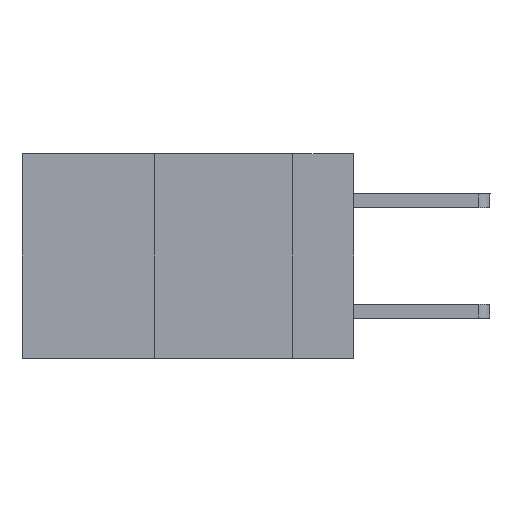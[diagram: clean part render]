
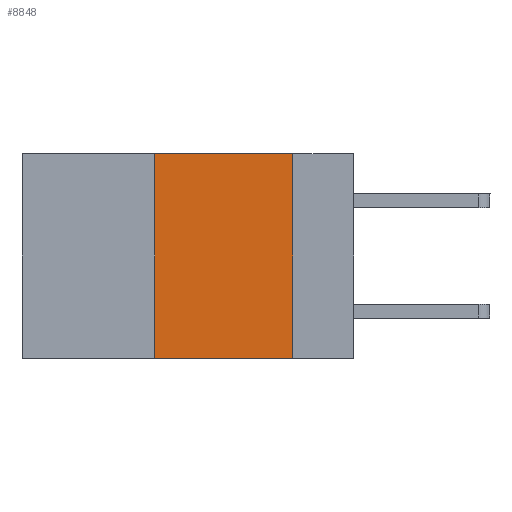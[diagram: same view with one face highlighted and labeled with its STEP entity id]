
A CAD part, left-side view. The second image highlights one B-rep face of the part: STEP entity #8848.
In plain terms, the highlighted planar face has unit normal (-1, 0, 0).
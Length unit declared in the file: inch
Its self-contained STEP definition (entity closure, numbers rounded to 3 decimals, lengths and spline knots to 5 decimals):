
#62 = VERTEX_POINT ( 'NONE', #6391 ) ;
#163 = DIRECTION ( 'NONE',  ( 0., 0., -1. ) ) ;
#187 = VECTOR ( 'NONE', #2608, 39.37008 ) ;
#459 = EDGE_LOOP ( 'NONE', ( #4697, #1227, #5542, #6564 ) ) ;
#501 = CARTESIAN_POINT ( 'NONE',  ( 0., 0.6, 0. ) ) ;
#928 = VERTEX_POINT ( 'NONE', #7984 ) ;
#1227 = ORIENTED_EDGE ( 'NONE', *, *, #7827, .F. ) ;
#1350 = VECTOR ( 'NONE', #163, 39.37008 ) ;
#1680 = CARTESIAN_POINT ( 'NONE',  ( 0., 0.6, -0.37 ) ) ;
#1956 = LINE ( 'NONE', #11112, #2784 ) ;
#2010 = CARTESIAN_POINT ( 'NONE',  ( 0., 0.36, 0. ) ) ;
#2598 = EDGE_CURVE ( 'NONE', #4305, #928, #8859, .T. ) ;
#2608 = DIRECTION ( 'NONE',  ( 0., -1., 0. ) ) ;
#2784 = VECTOR ( 'NONE', #6315, 39.37008 ) ;
#3645 = CARTESIAN_POINT ( 'NONE',  ( 0., 0.11, 0. ) ) ;
#3833 = PLANE ( 'NONE',  #4348 ) ;
#4013 = EDGE_CURVE ( 'NONE', #4519, #928, #6208, .T. ) ;
#4305 = VERTEX_POINT ( 'NONE', #5238 ) ;
#4348 = AXIS2_PLACEMENT_3D ( 'NONE', #501, #10348, #11075 ) ;
#4519 = VERTEX_POINT ( 'NONE', #9901 ) ;
#4697 = ORIENTED_EDGE ( 'NONE', *, *, #2598, .F. ) ;
#5238 = CARTESIAN_POINT ( 'NONE',  ( 0., 0.11, 0. ) ) ;
#5507 = DIRECTION ( 'NONE',  ( 0., 0., 1. ) ) ;
#5542 = ORIENTED_EDGE ( 'NONE', *, *, #11541, .F. ) ;
#6208 = LINE ( 'NONE', #1680, #187 ) ;
#6315 = DIRECTION ( 'NONE',  ( 0., -1., 0. ) ) ;
#6391 = CARTESIAN_POINT ( 'NONE',  ( 0., 0.36, 0. ) ) ;
#6564 = ORIENTED_EDGE ( 'NONE', *, *, #4013, .T. ) ;
#7827 = EDGE_CURVE ( 'NONE', #62, #4305, #1956, .T. ) ;
#7984 = CARTESIAN_POINT ( 'NONE',  ( 0., 0.11, -0.37 ) ) ;
#8111 = LINE ( 'NONE', #2010, #10087 ) ;
#8848 = ADVANCED_FACE ( 'NONE', ( #11132 ), #3833, .F. ) ;
#8859 = LINE ( 'NONE', #3645, #1350 ) ;
#9901 = CARTESIAN_POINT ( 'NONE',  ( 0., 0.36, -0.37 ) ) ;
#10087 = VECTOR ( 'NONE', #5507, 39.37008 ) ;
#10348 = DIRECTION ( 'NONE',  ( 1., 0., 0. ) ) ;
#11075 = DIRECTION ( 'NONE',  ( 0., 0., -1. ) ) ;
#11112 = CARTESIAN_POINT ( 'NONE',  ( 0., 0.6, 0. ) ) ;
#11132 = FACE_OUTER_BOUND ( 'NONE', #459, .T. ) ;
#11541 = EDGE_CURVE ( 'NONE', #4519, #62, #8111, .T. ) ;
